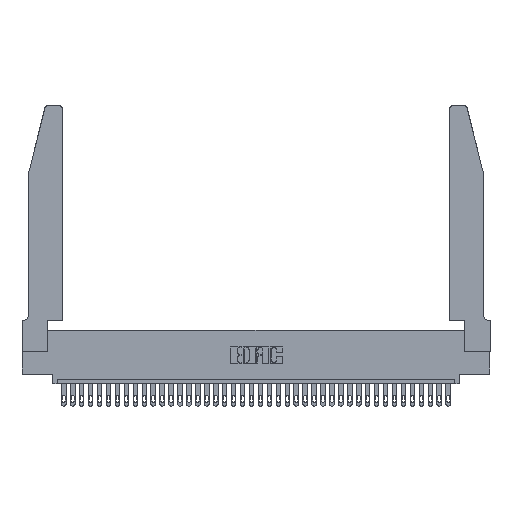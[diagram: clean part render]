
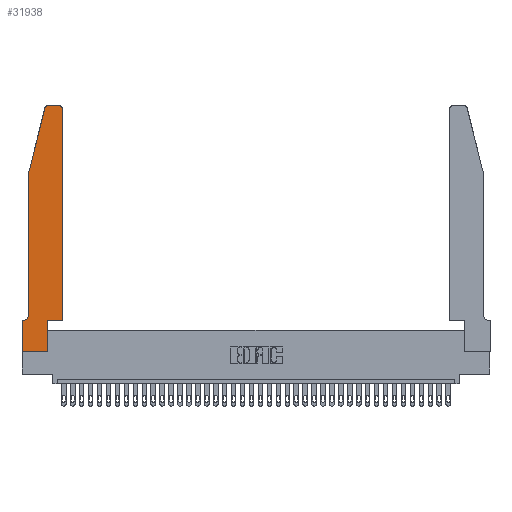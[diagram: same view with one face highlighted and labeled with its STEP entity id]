
A CAD part, top view. The second image highlights one B-rep face of the part: STEP entity #31938.
In plain terms, the highlighted planar face has unit normal (0, 0, 1).
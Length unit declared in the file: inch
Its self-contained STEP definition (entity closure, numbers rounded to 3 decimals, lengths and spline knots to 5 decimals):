
#230 = DIRECTION ( 'NONE',  ( 1., 0., 0. ) ) ;
#500 = EDGE_CURVE ( 'NONE', #16325, #30427, #30335, .T. ) ;
#614 = LINE ( 'NONE', #26302, #15112 ) ;
#829 = ORIENTED_EDGE ( 'NONE', *, *, #23036, .T. ) ;
#885 = LINE ( 'NONE', #15404, #16304 ) ;
#2055 = VERTEX_POINT ( 'NONE', #17421 ) ;
#2248 = EDGE_CURVE ( 'NONE', #26215, #23469, #22917, .T. ) ;
#2281 = AXIS2_PLACEMENT_3D ( 'NONE', #2315, #37623, #28531 ) ;
#2315 = CARTESIAN_POINT ( 'NONE',  ( 0.0055, 0.42, 0.37 ) ) ;
#3370 = FACE_OUTER_BOUND ( 'NONE', #35964, .T. ) ;
#3572 = PLANE ( 'NONE',  #23386 ) ;
#3760 = LINE ( 'NONE', #7206, #22358 ) ;
#6521 = CARTESIAN_POINT ( 'NONE',  ( 0.0755, 2., 0.37 ) ) ;
#6568 = EDGE_CURVE ( 'NONE', #37195, #29567, #13924, .T. ) ;
#6715 = DIRECTION ( 'NONE',  ( 1., 0., 0. ) ) ;
#7206 = CARTESIAN_POINT ( 'NONE',  ( 0.0755, 2., 0.37 ) ) ;
#7707 = CARTESIAN_POINT ( 'NONE',  ( 0.284, 2.75, 0.37 ) ) ;
#8003 = VECTOR ( 'NONE', #25923, 39.37008 ) ;
#8087 = CARTESIAN_POINT ( 'NONE',  ( 0.0755, 2., 0.37 ) ) ;
#8521 = LINE ( 'NONE', #26644, #33076 ) ;
#9169 = ORIENTED_EDGE ( 'NONE', *, *, #27072, .T. ) ;
#9554 = AXIS2_PLACEMENT_3D ( 'NONE', #18364, #33236, #15512 ) ;
#10623 = CARTESIAN_POINT ( 'NONE',  ( 0.2865, 0.35, 0.37 ) ) ;
#12676 = CARTESIAN_POINT ( 'NONE',  ( 0.25487, 2.72718, 0.37 ) ) ;
#12914 = ORIENTED_EDGE ( 'NONE', *, *, #30438, .T. ) ;
#12916 = DIRECTION ( 'NONE',  ( 0., -1., 0. ) ) ;
#13079 = DIRECTION ( 'NONE',  ( 0., -1., 0. ) ) ;
#13924 = LINE ( 'NONE', #37537, #8003 ) ;
#14255 = VECTOR ( 'NONE', #13079, 39.37008 ) ;
#14672 = CARTESIAN_POINT ( 'NONE',  ( 0.4505, 0.35, 0.37 ) ) ;
#14700 = VECTOR ( 'NONE', #37131, 39.37008 ) ;
#15112 = VECTOR ( 'NONE', #26546, 39.37008 ) ;
#15404 = CARTESIAN_POINT ( 'NONE',  ( 0., 0., 0.37 ) ) ;
#15421 = CARTESIAN_POINT ( 'NONE',  ( 0.0055, 0.35, 0.37 ) ) ;
#15451 = CARTESIAN_POINT ( 'NONE',  ( 0., 0., 0.37 ) ) ;
#15512 = DIRECTION ( 'NONE',  ( 1., 0., 0. ) ) ;
#15994 = ORIENTED_EDGE ( 'NONE', *, *, #30589, .T. ) ;
#16304 = VECTOR ( 'NONE', #29656, 39.37008 ) ;
#16323 = EDGE_CURVE ( 'NONE', #30427, #25840, #21560, .T. ) ;
#16325 = VERTEX_POINT ( 'NONE', #7707 ) ;
#17015 = CARTESIAN_POINT ( 'NONE',  ( 0.0755, 0.42, 0.37 ) ) ;
#17421 = CARTESIAN_POINT ( 'NONE',  ( 0.2865, 0.35, 0.37 ) ) ;
#17773 = CARTESIAN_POINT ( 'NONE',  ( 0., 0.35, 0.37 ) ) ;
#17895 = DIRECTION ( 'NONE',  ( -1., 0., 0. ) ) ;
#18134 = VERTEX_POINT ( 'NONE', #25499 ) ;
#18364 = CARTESIAN_POINT ( 'NONE',  ( 0.284, 2.72, 0.37 ) ) ;
#19009 = LINE ( 'NONE', #10623, #24456 ) ;
#19057 = CARTESIAN_POINT ( 'NONE',  ( 0., 0.35, 0.37 ) ) ;
#19889 = CIRCLE ( 'NONE', #34840, 0.03 ) ;
#21140 = VERTEX_POINT ( 'NONE', #15421 ) ;
#21286 = ORIENTED_EDGE ( 'NONE', *, *, #27759, .T. ) ;
#21463 = CARTESIAN_POINT ( 'NONE',  ( 0.4505, 2.72, 0.37 ) ) ;
#21560 = LINE ( 'NONE', #8087, #14700 ) ;
#22218 = VERTEX_POINT ( 'NONE', #31234 ) ;
#22358 = VECTOR ( 'NONE', #12916, 39.37008 ) ;
#22433 = DIRECTION ( 'NONE',  ( 0., 1., 0. ) ) ;
#22917 = LINE ( 'NONE', #15451, #14255 ) ;
#23036 = EDGE_CURVE ( 'NONE', #18134, #2055, #19009, .T. ) ;
#23386 = AXIS2_PLACEMENT_3D ( 'NONE', #17773, #29204, #230 ) ;
#23469 = VERTEX_POINT ( 'NONE', #29623 ) ;
#23868 = ORIENTED_EDGE ( 'NONE', *, *, #500, .T. ) ;
#23885 = ORIENTED_EDGE ( 'NONE', *, *, #26216, .T. ) ;
#24456 = VECTOR ( 'NONE', #22433, 39.37008 ) ;
#24519 = DIRECTION ( 'NONE',  ( 0., 0., 1. ) ) ;
#24547 = ORIENTED_EDGE ( 'NONE', *, *, #6568, .T. ) ;
#24781 = ORIENTED_EDGE ( 'NONE', *, *, #2248, .T. ) ;
#25261 = CARTESIAN_POINT ( 'NONE',  ( 0.4505, 0.35, 0.37 ) ) ;
#25499 = CARTESIAN_POINT ( 'NONE',  ( 0.2865, 0., 0.37 ) ) ;
#25840 = VERTEX_POINT ( 'NONE', #6521 ) ;
#25923 = DIRECTION ( 'NONE',  ( 0., 1., 0. ) ) ;
#26215 = VERTEX_POINT ( 'NONE', #19057 ) ;
#26216 = EDGE_CURVE ( 'NONE', #25840, #35811, #3760, .T. ) ;
#26302 = CARTESIAN_POINT ( 'NONE',  ( 0.0755, 0.35, 0.37 ) ) ;
#26546 = DIRECTION ( 'NONE',  ( -1., 0., 0. ) ) ;
#26644 = CARTESIAN_POINT ( 'NONE',  ( 0.2605, 2.75, 0.37 ) ) ;
#27058 = ORIENTED_EDGE ( 'NONE', *, *, #16323, .T. ) ;
#27072 = EDGE_CURVE ( 'NONE', #21140, #26215, #614, .T. ) ;
#27335 = LINE ( 'NONE', #25261, #36004 ) ;
#27540 = ORIENTED_EDGE ( 'NONE', *, *, #29364, .T. ) ;
#27759 = EDGE_CURVE ( 'NONE', #2055, #37195, #27335, .T. ) ;
#28531 = DIRECTION ( 'NONE',  ( -1., 0., 0. ) ) ;
#29204 = DIRECTION ( 'NONE',  ( 0., 0., 1. ) ) ;
#29364 = EDGE_CURVE ( 'NONE', #23469, #18134, #885, .T. ) ;
#29567 = VERTEX_POINT ( 'NONE', #21463 ) ;
#29623 = CARTESIAN_POINT ( 'NONE',  ( 0., 0., 0.37 ) ) ;
#29656 = DIRECTION ( 'NONE',  ( 1., 0., 0. ) ) ;
#30240 = EDGE_CURVE ( 'NONE', #22218, #16325, #8521, .T. ) ;
#30335 = CIRCLE ( 'NONE', #9554, 0.03 ) ;
#30427 = VERTEX_POINT ( 'NONE', #12676 ) ;
#30438 = EDGE_CURVE ( 'NONE', #29567, #22218, #19889, .T. ) ;
#30571 = ORIENTED_EDGE ( 'NONE', *, *, #30240, .T. ) ;
#30589 = EDGE_CURVE ( 'NONE', #35811, #21140, #37219, .T. ) ;
#31234 = CARTESIAN_POINT ( 'NONE',  ( 0.4205, 2.75, 0.37 ) ) ;
#31938 = ADVANCED_FACE ( 'NONE', ( #3370 ), #3572, .T. ) ;
#33076 = VECTOR ( 'NONE', #17895, 39.37008 ) ;
#33236 = DIRECTION ( 'NONE',  ( 0., 0., 1. ) ) ;
#34840 = AXIS2_PLACEMENT_3D ( 'NONE', #36229, #24519, #6715 ) ;
#35811 = VERTEX_POINT ( 'NONE', #17015 ) ;
#35964 = EDGE_LOOP ( 'NONE', ( #30571, #23868, #27058, #23885, #15994, #9169, #24781, #27540, #829, #21286, #24547, #12914 ) ) ;
#36004 = VECTOR ( 'NONE', #37020, 39.37008 ) ;
#36229 = CARTESIAN_POINT ( 'NONE',  ( 0.4205, 2.72, 0.37 ) ) ;
#37020 = DIRECTION ( 'NONE',  ( 1., 0., 0. ) ) ;
#37131 = DIRECTION ( 'NONE',  ( -0.239, -0.971, 0. ) ) ;
#37195 = VERTEX_POINT ( 'NONE', #14672 ) ;
#37219 = CIRCLE ( 'NONE', #2281, 0.07 ) ;
#37537 = CARTESIAN_POINT ( 'NONE',  ( 0.4505, 0.35, 0.37 ) ) ;
#37623 = DIRECTION ( 'NONE',  ( 0., 0., -1. ) ) ;
